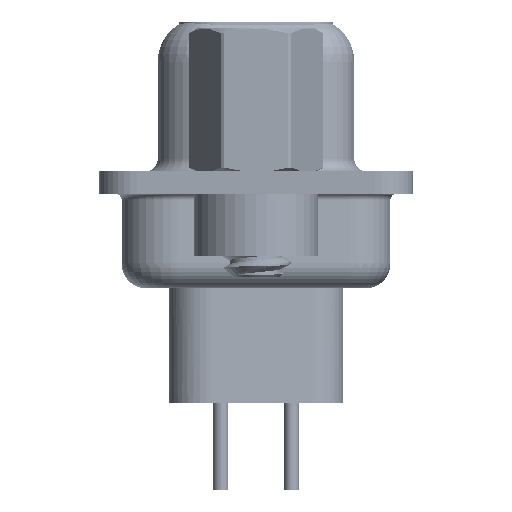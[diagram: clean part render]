
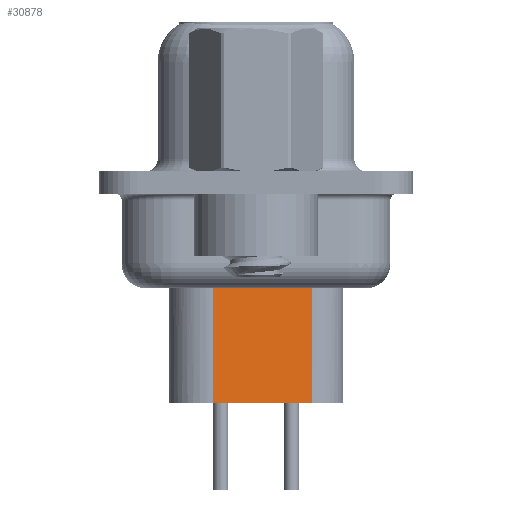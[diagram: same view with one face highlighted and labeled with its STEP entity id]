
A CAD part, left-side view. The second image highlights one B-rep face of the part: STEP entity #30878.
In plain terms, the highlighted planar face has unit normal (-0.985, -0.174, 0).
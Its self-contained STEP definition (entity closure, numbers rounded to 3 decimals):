
#266 = VECTOR ( 'NONE', #15130, 1000. ) ;
#989 = CARTESIAN_POINT ( 'NONE',  ( 4.524, 1.74, -8.85 ) ) ;
#1319 = ORIENTED_EDGE ( 'NONE', *, *, #12035, .T. ) ;
#2173 = VERTEX_POINT ( 'NONE', #5958 ) ;
#5958 = CARTESIAN_POINT ( 'NONE',  ( 4.524, 1.74, -8.85 ) ) ;
#6519 = DIRECTION ( 'NONE',  ( -0.174, 0.985, 0. ) ) ;
#7724 = ORIENTED_EDGE ( 'NONE', *, *, #10572, .T. ) ;
#7729 = CARTESIAN_POINT ( 'NONE',  ( 4.524, 1.74, -3.1 ) ) ;
#8097 = CARTESIAN_POINT ( 'NONE',  ( 5.229, -2.26, -8.85 ) ) ;
#9475 = VECTOR ( 'NONE', #23426, 1000. ) ;
#9710 = CARTESIAN_POINT ( 'NONE',  ( 4.524, 1.74, -3.1 ) ) ;
#9715 = CARTESIAN_POINT ( 'NONE',  ( 4.353, 2.709, -3.975 ) ) ;
#10572 = EDGE_CURVE ( 'NONE', #33743, #2173, #21373, .T. ) ;
#12035 = EDGE_CURVE ( 'NONE', #18362, #33743, #29285, .T. ) ;
#13770 = EDGE_CURVE ( 'NONE', #29239, #2173, #29626, .T. ) ;
#15130 = DIRECTION ( 'NONE',  ( 0., 0., -1. ) ) ;
#15845 = CARTESIAN_POINT ( 'NONE',  ( 5.229, -2.26, -3.1 ) ) ;
#16050 = CARTESIAN_POINT ( 'NONE',  ( 5.229, -2.26, -3.975 ) ) ;
#18362 = VERTEX_POINT ( 'NONE', #16050 ) ;
#18695 = LINE ( 'NONE', #15845, #266 ) ;
#19200 = DIRECTION ( 'NONE',  ( 0.174, -0.985, 0. ) ) ;
#19653 = AXIS2_PLACEMENT_3D ( 'NONE', #7729, #24309, #19200 ) ;
#20399 = EDGE_LOOP ( 'NONE', ( #35663, #1319, #7724, #29996 ) ) ;
#21373 = LINE ( 'NONE', #9710, #33072 ) ;
#22034 = FACE_OUTER_BOUND ( 'NONE', #20399, .T. ) ;
#23426 = DIRECTION ( 'NONE',  ( -0.174, 0.985, 0. ) ) ;
#24309 = DIRECTION ( 'NONE',  ( -0.985, -0.174, 0. ) ) ;
#27350 = EDGE_CURVE ( 'NONE', #18362, #29239, #18695, .T. ) ;
#29239 = VERTEX_POINT ( 'NONE', #8097 ) ;
#29285 = LINE ( 'NONE', #9715, #31048 ) ;
#29626 = LINE ( 'NONE', #989, #9475 ) ;
#29996 = ORIENTED_EDGE ( 'NONE', *, *, #13770, .F. ) ;
#30878 = ADVANCED_FACE ( 'NONE', ( #22034 ), #33506, .T. ) ;
#31048 = VECTOR ( 'NONE', #6519, 1000. ) ;
#33072 = VECTOR ( 'NONE', #35287, 1000. ) ;
#33458 = CARTESIAN_POINT ( 'NONE',  ( 4.524, 1.74, -3.975 ) ) ;
#33506 = PLANE ( 'NONE',  #19653 ) ;
#33743 = VERTEX_POINT ( 'NONE', #33458 ) ;
#35287 = DIRECTION ( 'NONE',  ( 0., 0., -1. ) ) ;
#35663 = ORIENTED_EDGE ( 'NONE', *, *, #27350, .F. ) ;
